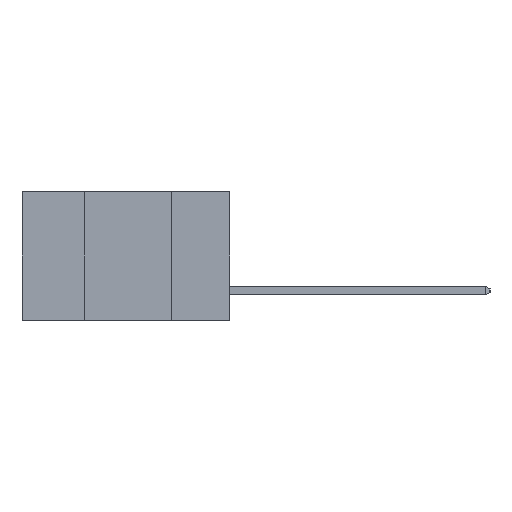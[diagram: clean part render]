
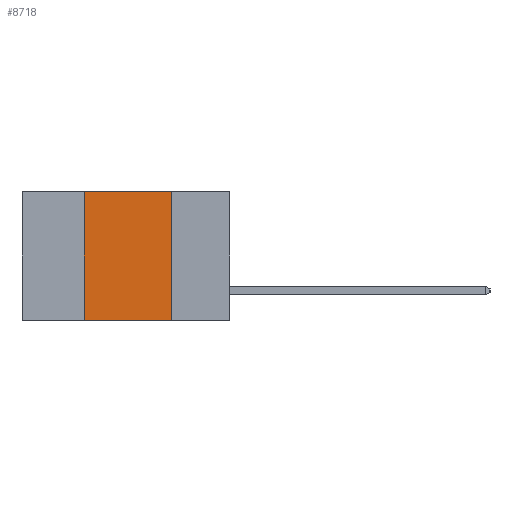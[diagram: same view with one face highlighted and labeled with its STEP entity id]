
A CAD part, left-side view. The second image highlights one B-rep face of the part: STEP entity #8718.
In plain terms, the highlighted planar face has unit normal (-1, 0, 0).
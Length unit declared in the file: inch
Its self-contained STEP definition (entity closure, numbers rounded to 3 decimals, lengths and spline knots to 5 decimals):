
#195 = DIRECTION ( 'NONE',  ( 0., -1., 0. ) ) ;
#2524 = ORIENTED_EDGE ( 'NONE', *, *, #2898, .F. ) ;
#2898 = EDGE_CURVE ( 'NONE', #5590, #4682, #6407, .T. ) ;
#3077 = EDGE_LOOP ( 'NONE', ( #2524, #7016, #6668, #5676 ) ) ;
#3154 = CARTESIAN_POINT ( 'NONE',  ( 0., 0.6, 0. ) ) ;
#3318 = LINE ( 'NONE', #10899, #7453 ) ;
#3608 = VERTEX_POINT ( 'NONE', #3966 ) ;
#3704 = EDGE_CURVE ( 'NONE', #9185, #5590, #11239, .T. ) ;
#3966 = CARTESIAN_POINT ( 'NONE',  ( 0., 0.42, -0.37 ) ) ;
#4524 = DIRECTION ( 'NONE',  ( 1., 0., 0. ) ) ;
#4682 = VERTEX_POINT ( 'NONE', #7383 ) ;
#5590 = VERTEX_POINT ( 'NONE', #5710 ) ;
#5671 = DIRECTION ( 'NONE',  ( 0., 0., 1. ) ) ;
#5676 = ORIENTED_EDGE ( 'NONE', *, *, #11878, .T. ) ;
#5710 = CARTESIAN_POINT ( 'NONE',  ( 0., 0.17, 0. ) ) ;
#6383 = CARTESIAN_POINT ( 'NONE',  ( 0., 0.42, 0. ) ) ;
#6387 = DIRECTION ( 'NONE',  ( 0., 0., -1. ) ) ;
#6407 = LINE ( 'NONE', #9558, #8746 ) ;
#6668 = ORIENTED_EDGE ( 'NONE', *, *, #10546, .F. ) ;
#6906 = VECTOR ( 'NONE', #12801, 39.37008 ) ;
#7016 = ORIENTED_EDGE ( 'NONE', *, *, #3704, .F. ) ;
#7383 = CARTESIAN_POINT ( 'NONE',  ( 0., 0.17, -0.37 ) ) ;
#7453 = VECTOR ( 'NONE', #5671, 39.37008 ) ;
#7612 = CARTESIAN_POINT ( 'NONE',  ( 0., 0.6, 0. ) ) ;
#7706 = DIRECTION ( 'NONE',  ( 0., 0., -1. ) ) ;
#7841 = FACE_OUTER_BOUND ( 'NONE', #3077, .T. ) ;
#8718 = ADVANCED_FACE ( 'NONE', ( #7841 ), #11928, .F. ) ;
#8746 = VECTOR ( 'NONE', #6387, 39.37008 ) ;
#9185 = VERTEX_POINT ( 'NONE', #6383 ) ;
#9258 = LINE ( 'NONE', #11696, #11625 ) ;
#9558 = CARTESIAN_POINT ( 'NONE',  ( 0., 0.17, -0.37 ) ) ;
#10546 = EDGE_CURVE ( 'NONE', #3608, #9185, #3318, .T. ) ;
#10899 = CARTESIAN_POINT ( 'NONE',  ( 0., 0.42, -0.37 ) ) ;
#11139 = AXIS2_PLACEMENT_3D ( 'NONE', #7612, #4524, #7706 ) ;
#11239 = LINE ( 'NONE', #3154, #6906 ) ;
#11625 = VECTOR ( 'NONE', #195, 39.37008 ) ;
#11696 = CARTESIAN_POINT ( 'NONE',  ( 0., 0.6, -0.37 ) ) ;
#11878 = EDGE_CURVE ( 'NONE', #3608, #4682, #9258, .T. ) ;
#11928 = PLANE ( 'NONE',  #11139 ) ;
#12801 = DIRECTION ( 'NONE',  ( 0., -1., 0. ) ) ;
